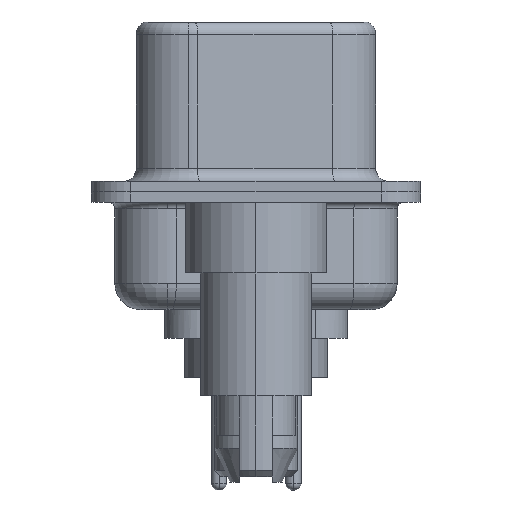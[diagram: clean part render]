
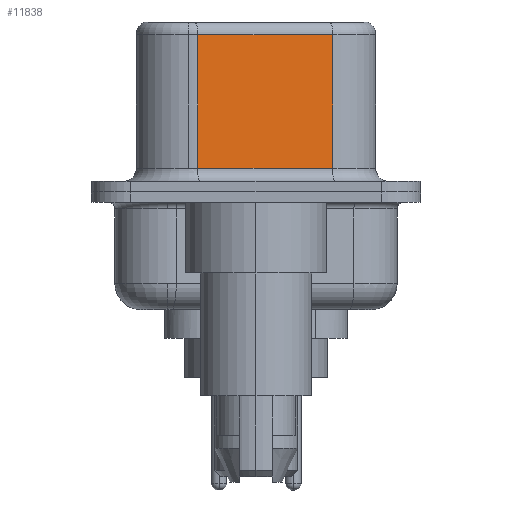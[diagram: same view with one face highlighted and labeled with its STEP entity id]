
A CAD part, left-side view. The second image highlights one B-rep face of the part: STEP entity #11838.
In plain terms, the highlighted planar face has unit normal (-0.985, -0.174, 0).
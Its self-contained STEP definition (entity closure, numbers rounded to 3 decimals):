
#491 = CARTESIAN_POINT ( 'NONE',  ( 4.585, -2.927, 6.02 ) ) ;
#1223 = VECTOR ( 'NONE', #3291, 1000. ) ;
#1575 = CARTESIAN_POINT ( 'NONE',  ( 4.585, -2.927, 6.52 ) ) ;
#1683 = VERTEX_POINT ( 'NONE', #10719 ) ;
#2045 = LINE ( 'NONE', #7754, #11358 ) ;
#2416 = DIRECTION ( 'NONE',  ( 0.174, -0.985, 0. ) ) ;
#3287 = DIRECTION ( 'NONE',  ( 0., 0., -1. ) ) ;
#3291 = DIRECTION ( 'NONE',  ( -0.174, 0.985, 0. ) ) ;
#4426 = VERTEX_POINT ( 'NONE', #13298 ) ;
#4468 = AXIS2_PLACEMENT_3D ( 'NONE', #15992, #11369, #8221 ) ;
#5621 = EDGE_LOOP ( 'NONE', ( #13218, #12879, #7028, #11503 ) ) ;
#5820 = LINE ( 'NONE', #14935, #18799 ) ;
#6524 = VERTEX_POINT ( 'NONE', #13440 ) ;
#6692 = LINE ( 'NONE', #1575, #18677 ) ;
#7028 = ORIENTED_EDGE ( 'NONE', *, *, #18738, .T. ) ;
#7421 = EDGE_CURVE ( 'NONE', #16716, #6524, #6692, .T. ) ;
#7754 = CARTESIAN_POINT ( 'NONE',  ( 3.675, 2.233, 6.52 ) ) ;
#8221 = DIRECTION ( 'NONE',  ( -0.174, 0.985, 0. ) ) ;
#9260 = DIRECTION ( 'NONE',  ( 0., 0., -1. ) ) ;
#10719 = CARTESIAN_POINT ( 'NONE',  ( 3.675, 2.233, 6.02 ) ) ;
#11358 = VECTOR ( 'NONE', #3287, 1000. ) ;
#11369 = DIRECTION ( 'NONE',  ( 0.985, 0.174, 0. ) ) ;
#11414 = EDGE_CURVE ( 'NONE', #4426, #6524, #5820, .T. ) ;
#11503 = ORIENTED_EDGE ( 'NONE', *, *, #11414, .T. ) ;
#11838 = ADVANCED_FACE ( 'NONE', ( #19048 ), #16126, .F. ) ;
#12879 = ORIENTED_EDGE ( 'NONE', *, *, #14452, .T. ) ;
#13218 = ORIENTED_EDGE ( 'NONE', *, *, #7421, .F. ) ;
#13298 = CARTESIAN_POINT ( 'NONE',  ( 3.675, 2.233, 0.9 ) ) ;
#13440 = CARTESIAN_POINT ( 'NONE',  ( 4.585, -2.927, 0.9 ) ) ;
#14038 = CARTESIAN_POINT ( 'NONE',  ( 4.585, -2.927, 6.02 ) ) ;
#14452 = EDGE_CURVE ( 'NONE', #16716, #1683, #17387, .T. ) ;
#14935 = CARTESIAN_POINT ( 'NONE',  ( 4.585, -2.927, 0.9 ) ) ;
#15992 = CARTESIAN_POINT ( 'NONE',  ( 4.585, -2.927, 6.52 ) ) ;
#16126 = PLANE ( 'NONE',  #4468 ) ;
#16716 = VERTEX_POINT ( 'NONE', #491 ) ;
#17387 = LINE ( 'NONE', #14038, #1223 ) ;
#18677 = VECTOR ( 'NONE', #9260, 1000. ) ;
#18738 = EDGE_CURVE ( 'NONE', #1683, #4426, #2045, .T. ) ;
#18799 = VECTOR ( 'NONE', #2416, 1000. ) ;
#19048 = FACE_OUTER_BOUND ( 'NONE', #5621, .T. ) ;
